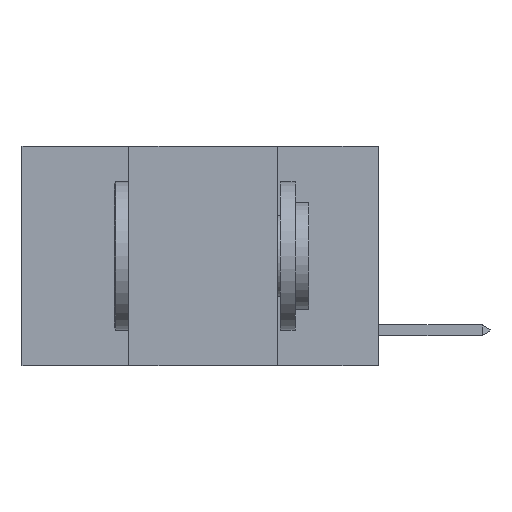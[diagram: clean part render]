
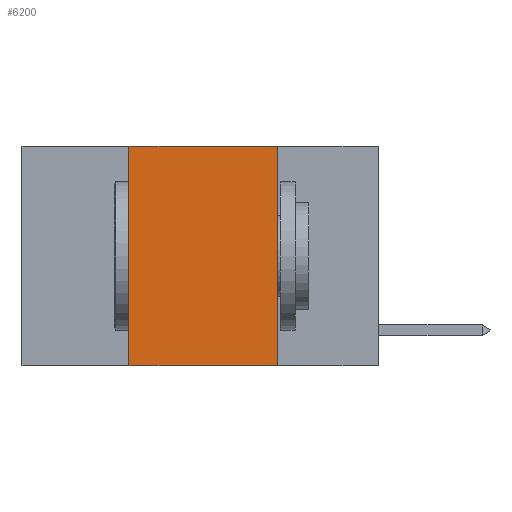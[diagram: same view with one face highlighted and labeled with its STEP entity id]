
A CAD part, left-side view. The second image highlights one B-rep face of the part: STEP entity #6200.
In plain terms, the highlighted planar face has unit normal (-1, 0, 0).
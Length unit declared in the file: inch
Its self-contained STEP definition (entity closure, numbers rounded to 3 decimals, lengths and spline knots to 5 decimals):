
#147 = EDGE_LOOP ( 'NONE', ( #495, #724, #6031, #6511 ) ) ;
#314 = VECTOR ( 'NONE', #7625, 39.37008 ) ;
#495 = ORIENTED_EDGE ( 'NONE', *, *, #2970, .F. ) ;
#724 = ORIENTED_EDGE ( 'NONE', *, *, #5009, .F. ) ;
#819 = LINE ( 'NONE', #8490, #314 ) ;
#1141 = DIRECTION ( 'NONE',  ( 1., 0., 0. ) ) ;
#1631 = VERTEX_POINT ( 'NONE', #8681 ) ;
#1929 = PLANE ( 'NONE',  #3459 ) ;
#2173 = DIRECTION ( 'NONE',  ( 0., 0., 1. ) ) ;
#2582 = CARTESIAN_POINT ( 'NONE',  ( 0., 0.6, -0.37 ) ) ;
#2781 = VECTOR ( 'NONE', #9062, 39.37008 ) ;
#2819 = CARTESIAN_POINT ( 'NONE',  ( 0., 0.17, -0.37 ) ) ;
#2970 = EDGE_CURVE ( 'NONE', #1631, #5889, #819, .T. ) ;
#3306 = LINE ( 'NONE', #7072, #3701 ) ;
#3459 = AXIS2_PLACEMENT_3D ( 'NONE', #7514, #1141, #9088 ) ;
#3701 = VECTOR ( 'NONE', #2173, 39.37008 ) ;
#4114 = LINE ( 'NONE', #10180, #5452 ) ;
#5009 = EDGE_CURVE ( 'NONE', #5468, #1631, #4114, .T. ) ;
#5318 = FACE_OUTER_BOUND ( 'NONE', #147, .T. ) ;
#5452 = VECTOR ( 'NONE', #7002, 39.37008 ) ;
#5468 = VERTEX_POINT ( 'NONE', #9714 ) ;
#5765 = VERTEX_POINT ( 'NONE', #10463 ) ;
#5889 = VERTEX_POINT ( 'NONE', #2819 ) ;
#6031 = ORIENTED_EDGE ( 'NONE', *, *, #9676, .F. ) ;
#6200 = ADVANCED_FACE ( 'NONE', ( #5318 ), #1929, .F. ) ;
#6511 = ORIENTED_EDGE ( 'NONE', *, *, #9807, .T. ) ;
#7002 = DIRECTION ( 'NONE',  ( 0., -1., 0. ) ) ;
#7072 = CARTESIAN_POINT ( 'NONE',  ( 0., 0.42, 0. ) ) ;
#7514 = CARTESIAN_POINT ( 'NONE',  ( 0., 0.6, 0. ) ) ;
#7625 = DIRECTION ( 'NONE',  ( 0., 0., -1. ) ) ;
#8415 = LINE ( 'NONE', #2582, #2781 ) ;
#8490 = CARTESIAN_POINT ( 'NONE',  ( 0., 0.17, 0. ) ) ;
#8681 = CARTESIAN_POINT ( 'NONE',  ( 0., 0.17, 0. ) ) ;
#9062 = DIRECTION ( 'NONE',  ( 0., -1., 0. ) ) ;
#9088 = DIRECTION ( 'NONE',  ( 0., 0., -1. ) ) ;
#9676 = EDGE_CURVE ( 'NONE', #5765, #5468, #3306, .T. ) ;
#9714 = CARTESIAN_POINT ( 'NONE',  ( 0., 0.42, 0. ) ) ;
#9807 = EDGE_CURVE ( 'NONE', #5765, #5889, #8415, .T. ) ;
#10180 = CARTESIAN_POINT ( 'NONE',  ( 0., 0.6, 0. ) ) ;
#10463 = CARTESIAN_POINT ( 'NONE',  ( 0., 0.42, -0.37 ) ) ;
